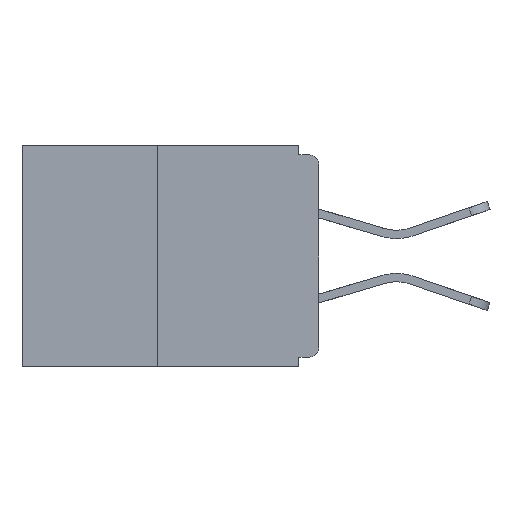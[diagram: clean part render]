
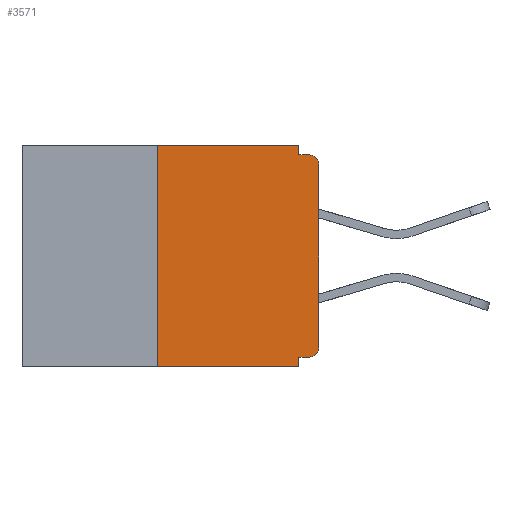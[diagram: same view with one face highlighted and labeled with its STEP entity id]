
A CAD part, left-side view. The second image highlights one B-rep face of the part: STEP entity #3571.
In plain terms, the highlighted planar face has unit normal (-1, 0, 0).
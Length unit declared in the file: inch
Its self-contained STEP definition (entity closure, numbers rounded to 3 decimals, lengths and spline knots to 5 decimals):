
#352 = EDGE_CURVE ( 'NONE', #2817, #9573, #10820, .T. ) ;
#656 = EDGE_CURVE ( 'NONE', #5261, #1344, #3766, .T. ) ;
#1000 = LINE ( 'NONE', #10064, #6888 ) ;
#1123 = LINE ( 'NONE', #9420, #9050 ) ;
#1152 = VERTEX_POINT ( 'NONE', #1874 ) ;
#1195 = EDGE_CURVE ( 'NONE', #10649, #9017, #7328, .T. ) ;
#1344 = VERTEX_POINT ( 'NONE', #8492 ) ;
#1487 = EDGE_CURVE ( 'NONE', #3511, #11304, #6741, .T. ) ;
#1559 = DIRECTION ( 'NONE',  ( -1., 0., 0. ) ) ;
#1633 = CARTESIAN_POINT ( 'NONE',  ( 0., 0.015, -0.03 ) ) ;
#1685 = ORIENTED_EDGE ( 'NONE', *, *, #4499, .F. ) ;
#1765 = ORIENTED_EDGE ( 'NONE', *, *, #7598, .F. ) ;
#1779 = EDGE_CURVE ( 'NONE', #7564, #1344, #1000, .T. ) ;
#1864 = FACE_OUTER_BOUND ( 'NONE', #8129, .T. ) ;
#1874 = CARTESIAN_POINT ( 'NONE',  ( 0., 0.031, -0.328 ) ) ;
#2000 = CARTESIAN_POINT ( 'NONE',  ( 0., 0., -0.313 ) ) ;
#2029 = DIRECTION ( 'NONE',  ( 0., 0., -1. ) ) ;
#2033 = DIRECTION ( 'NONE',  ( 0., -1., 0. ) ) ;
#2817 = VERTEX_POINT ( 'NONE', #8318 ) ;
#3296 = ORIENTED_EDGE ( 'NONE', *, *, #5320, .T. ) ;
#3368 = DIRECTION ( 'NONE',  ( 0., 0., -1. ) ) ;
#3498 = AXIS2_PLACEMENT_3D ( 'NONE', #6490, #3868, #2029 ) ;
#3511 = VERTEX_POINT ( 'NONE', #11757 ) ;
#3528 = ORIENTED_EDGE ( 'NONE', *, *, #4316, .F. ) ;
#3571 = ADVANCED_FACE ( 'NONE', ( #1864 ), #8908, .F. ) ;
#3591 = DIRECTION ( 'NONE',  ( 0., -1., 0. ) ) ;
#3766 = CIRCLE ( 'NONE', #6531, 0.015 ) ;
#3815 = EDGE_CURVE ( 'NONE', #10649, #1152, #8033, .T. ) ;
#3868 = DIRECTION ( 'NONE',  ( -1., 0., 0. ) ) ;
#3890 = DIRECTION ( 'NONE',  ( 0., 0., 1. ) ) ;
#4242 = AXIS2_PLACEMENT_3D ( 'NONE', #6239, #10451, #5843 ) ;
#4316 = EDGE_CURVE ( 'NONE', #9573, #7564, #1123, .T. ) ;
#4491 = LINE ( 'NONE', #4897, #7659 ) ;
#4499 = EDGE_CURVE ( 'NONE', #1152, #11304, #7445, .T. ) ;
#4897 = CARTESIAN_POINT ( 'NONE',  ( 0., 0.25, 0. ) ) ;
#5222 = ORIENTED_EDGE ( 'NONE', *, *, #656, .T. ) ;
#5261 = VERTEX_POINT ( 'NONE', #5970 ) ;
#5298 = VECTOR ( 'NONE', #9316, 39.37008 ) ;
#5305 = CARTESIAN_POINT ( 'NONE',  ( 0., 0.031, 0. ) ) ;
#5320 = EDGE_CURVE ( 'NONE', #9017, #5261, #8166, .T. ) ;
#5639 = ORIENTED_EDGE ( 'NONE', *, *, #1779, .F. ) ;
#5843 = DIRECTION ( 'NONE',  ( 0., 0., -1. ) ) ;
#5970 = CARTESIAN_POINT ( 'NONE',  ( 0., 0., -0.03 ) ) ;
#6239 = CARTESIAN_POINT ( 'NONE',  ( 0., 0.46, 0. ) ) ;
#6490 = CARTESIAN_POINT ( 'NONE',  ( 0., 0.015, -0.313 ) ) ;
#6531 = AXIS2_PLACEMENT_3D ( 'NONE', #1633, #1559, #3368 ) ;
#6741 = LINE ( 'NONE', #11196, #11932 ) ;
#6888 = VECTOR ( 'NONE', #9409, 39.37008 ) ;
#7280 = CARTESIAN_POINT ( 'NONE',  ( 0., 0.46, 0. ) ) ;
#7328 = CIRCLE ( 'NONE', #3498, 0.015 ) ;
#7396 = CARTESIAN_POINT ( 'NONE',  ( 0., 0.031, -0.343 ) ) ;
#7445 = LINE ( 'NONE', #7396, #5298 ) ;
#7564 = VERTEX_POINT ( 'NONE', #8618 ) ;
#7598 = EDGE_CURVE ( 'NONE', #3511, #2817, #4491, .T. ) ;
#7659 = VECTOR ( 'NONE', #3890, 39.37008 ) ;
#8033 = LINE ( 'NONE', #9182, #10179 ) ;
#8129 = EDGE_LOOP ( 'NONE', ( #11518, #1765, #8942, #1685, #10303, #8860, #3296, #5222, #5639, #3528 ) ) ;
#8166 = LINE ( 'NONE', #11657, #8452 ) ;
#8219 = VECTOR ( 'NONE', #3591, 39.37008 ) ;
#8288 = CARTESIAN_POINT ( 'NONE',  ( 0., 0.031, -0.343 ) ) ;
#8318 = CARTESIAN_POINT ( 'NONE',  ( 0., 0.25, 0. ) ) ;
#8452 = VECTOR ( 'NONE', #8965, 39.37008 ) ;
#8492 = CARTESIAN_POINT ( 'NONE',  ( 0., 0.015, -0.015 ) ) ;
#8618 = CARTESIAN_POINT ( 'NONE',  ( 0., 0.031, -0.015 ) ) ;
#8860 = ORIENTED_EDGE ( 'NONE', *, *, #1195, .T. ) ;
#8908 = PLANE ( 'NONE',  #4242 ) ;
#8942 = ORIENTED_EDGE ( 'NONE', *, *, #1487, .T. ) ;
#8965 = DIRECTION ( 'NONE',  ( 0., 0., 1. ) ) ;
#9017 = VERTEX_POINT ( 'NONE', #2000 ) ;
#9050 = VECTOR ( 'NONE', #10450, 39.37008 ) ;
#9182 = CARTESIAN_POINT ( 'NONE',  ( 0., 0., -0.328 ) ) ;
#9316 = DIRECTION ( 'NONE',  ( 0., 0., -1. ) ) ;
#9409 = DIRECTION ( 'NONE',  ( 0., -1., 0. ) ) ;
#9420 = CARTESIAN_POINT ( 'NONE',  ( 0., 0.031, 0. ) ) ;
#9573 = VERTEX_POINT ( 'NONE', #5305 ) ;
#9998 = DIRECTION ( 'NONE',  ( 0., 1., 0. ) ) ;
#10064 = CARTESIAN_POINT ( 'NONE',  ( 0., 0., -0.015 ) ) ;
#10179 = VECTOR ( 'NONE', #9998, 39.37008 ) ;
#10303 = ORIENTED_EDGE ( 'NONE', *, *, #3815, .F. ) ;
#10450 = DIRECTION ( 'NONE',  ( 0., 0., -1. ) ) ;
#10451 = DIRECTION ( 'NONE',  ( 1., 0., 0. ) ) ;
#10649 = VERTEX_POINT ( 'NONE', #11477 ) ;
#10820 = LINE ( 'NONE', #7280, #8219 ) ;
#11196 = CARTESIAN_POINT ( 'NONE',  ( 0., 0.46, -0.343 ) ) ;
#11304 = VERTEX_POINT ( 'NONE', #8288 ) ;
#11477 = CARTESIAN_POINT ( 'NONE',  ( 0., 0.015, -0.328 ) ) ;
#11518 = ORIENTED_EDGE ( 'NONE', *, *, #352, .F. ) ;
#11657 = CARTESIAN_POINT ( 'NONE',  ( 0., 0., 0. ) ) ;
#11757 = CARTESIAN_POINT ( 'NONE',  ( 0., 0.25, -0.343 ) ) ;
#11932 = VECTOR ( 'NONE', #2033, 39.37008 ) ;
